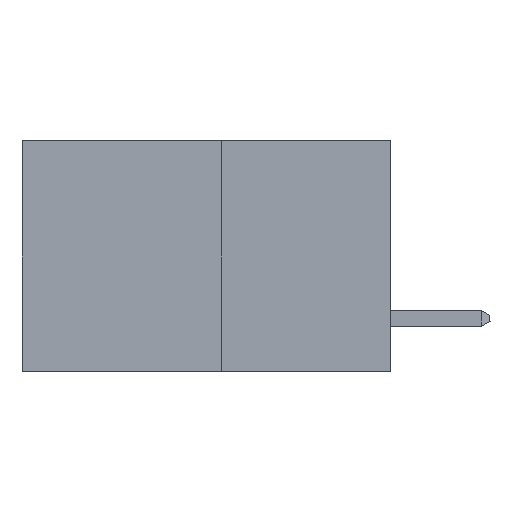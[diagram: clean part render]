
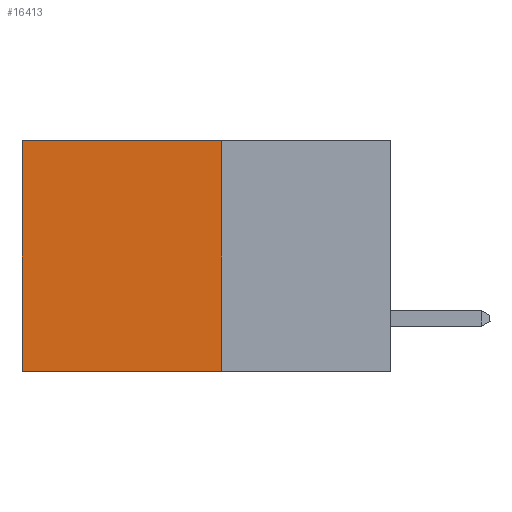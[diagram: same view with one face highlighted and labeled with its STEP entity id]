
A CAD part, left-side view. The second image highlights one B-rep face of the part: STEP entity #16413.
In plain terms, the highlighted planar face has unit normal (-1, 0, 0).
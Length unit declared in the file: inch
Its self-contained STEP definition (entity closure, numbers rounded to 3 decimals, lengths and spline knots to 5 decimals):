
#2148 = VERTEX_POINT ( 'NONE', #9647 ) ;
#2935 = CARTESIAN_POINT ( 'NONE',  ( 0.277, 0.27, 0. ) ) ;
#3226 = CARTESIAN_POINT ( 'NONE',  ( 0.277, 0.27, -0.37 ) ) ;
#4256 = VERTEX_POINT ( 'NONE', #2935 ) ;
#6092 = VECTOR ( 'NONE', #18828, 39.37008 ) ;
#6615 = ORIENTED_EDGE ( 'NONE', *, *, #16492, .F. ) ;
#6740 = EDGE_LOOP ( 'NONE', ( #6817, #21235, #6615, #23885 ) ) ;
#6817 = ORIENTED_EDGE ( 'NONE', *, *, #9164, .T. ) ;
#7525 = CARTESIAN_POINT ( 'NONE',  ( 0.277, 0.59, -0.37 ) ) ;
#7705 = DIRECTION ( 'NONE',  ( 0., 0., -1. ) ) ;
#8175 = EDGE_CURVE ( 'NONE', #21520, #2148, #16965, .T. ) ;
#9007 = DIRECTION ( 'NONE',  ( 0., 0., -1. ) ) ;
#9164 = EDGE_CURVE ( 'NONE', #16572, #2148, #15090, .T. ) ;
#9647 = CARTESIAN_POINT ( 'NONE',  ( 0.277, 0.59, -0.37 ) ) ;
#11335 = LINE ( 'NONE', #3226, #6092 ) ;
#11920 = CARTESIAN_POINT ( 'NONE',  ( 0.277, 0.27, 0. ) ) ;
#13859 = DIRECTION ( 'NONE',  ( 0., 1., 0. ) ) ;
#15090 = LINE ( 'NONE', #7525, #15682 ) ;
#15388 = EDGE_CURVE ( 'NONE', #4256, #16572, #17430, .T. ) ;
#15682 = VECTOR ( 'NONE', #7705, 39.37008 ) ;
#16413 = ADVANCED_FACE ( 'NONE', ( #17683 ), #16618, .F. ) ;
#16492 = EDGE_CURVE ( 'NONE', #4256, #21520, #11335, .T. ) ;
#16572 = VERTEX_POINT ( 'NONE', #17108 ) ;
#16618 = PLANE ( 'NONE',  #17421 ) ;
#16823 = VECTOR ( 'NONE', #13859, 39.37008 ) ;
#16965 = LINE ( 'NONE', #18821, #22725 ) ;
#17108 = CARTESIAN_POINT ( 'NONE',  ( 0.277, 0.59, 0. ) ) ;
#17421 = AXIS2_PLACEMENT_3D ( 'NONE', #18651, #20598, #9007 ) ;
#17430 = LINE ( 'NONE', #11920, #16823 ) ;
#17683 = FACE_OUTER_BOUND ( 'NONE', #6740, .T. ) ;
#18625 = DIRECTION ( 'NONE',  ( 0., 1., 0. ) ) ;
#18651 = CARTESIAN_POINT ( 'NONE',  ( 0.277, 0.27, -0.37 ) ) ;
#18821 = CARTESIAN_POINT ( 'NONE',  ( 0.277, 0.27, -0.37 ) ) ;
#18828 = DIRECTION ( 'NONE',  ( 0., 0., -1. ) ) ;
#20598 = DIRECTION ( 'NONE',  ( 1., 0., 0. ) ) ;
#21235 = ORIENTED_EDGE ( 'NONE', *, *, #8175, .F. ) ;
#21520 = VERTEX_POINT ( 'NONE', #22220 ) ;
#22220 = CARTESIAN_POINT ( 'NONE',  ( 0.277, 0.27, -0.37 ) ) ;
#22725 = VECTOR ( 'NONE', #18625, 39.37008 ) ;
#23885 = ORIENTED_EDGE ( 'NONE', *, *, #15388, .T. ) ;
